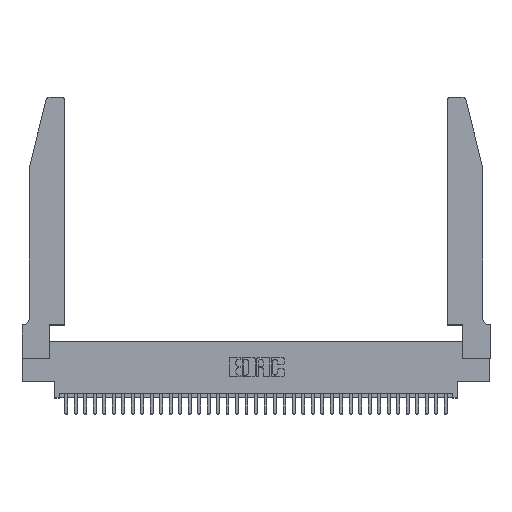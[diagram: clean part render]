
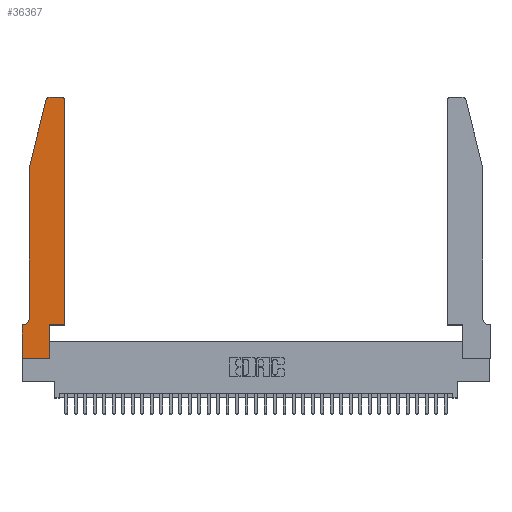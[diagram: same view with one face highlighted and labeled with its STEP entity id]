
A CAD part, top view. The second image highlights one B-rep face of the part: STEP entity #36367.
In plain terms, the highlighted planar face has unit normal (0, 0, 1).
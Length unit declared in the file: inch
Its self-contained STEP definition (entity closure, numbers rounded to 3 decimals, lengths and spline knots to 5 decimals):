
#19 = EDGE_LOOP ( 'NONE', ( #13343, #34293, #35894, #194, #32625, #27486, #5706, #4001, #19048, #23424, #12861, #13882 ) ) ;
#194 = ORIENTED_EDGE ( 'NONE', *, *, #6207, .T. ) ;
#359 = CIRCLE ( 'NONE', #16648, 0.03 ) ;
#873 = VECTOR ( 'NONE', #36660, 39.37008 ) ;
#877 = CARTESIAN_POINT ( 'NONE',  ( 0.4505, 0.35, 0.37 ) ) ;
#1088 = CARTESIAN_POINT ( 'NONE',  ( 0., 0.35, 0.37 ) ) ;
#2234 = VERTEX_POINT ( 'NONE', #5444 ) ;
#2669 = VECTOR ( 'NONE', #34483, 39.37008 ) ;
#3150 = CARTESIAN_POINT ( 'NONE',  ( 0., 0., 0.37 ) ) ;
#3686 = DIRECTION ( 'NONE',  ( 0., 1., 0. ) ) ;
#3735 = CARTESIAN_POINT ( 'NONE',  ( 0.0755, 0.42, 0.37 ) ) ;
#4001 = ORIENTED_EDGE ( 'NONE', *, *, #28637, .T. ) ;
#4124 = EDGE_CURVE ( 'NONE', #32632, #2234, #359, .T. ) ;
#4449 = CARTESIAN_POINT ( 'NONE',  ( 0.4505, 0.35, 0.37 ) ) ;
#4918 = VERTEX_POINT ( 'NONE', #33622 ) ;
#5171 = VERTEX_POINT ( 'NONE', #34726 ) ;
#5190 = VECTOR ( 'NONE', #11448, 39.37008 ) ;
#5444 = CARTESIAN_POINT ( 'NONE',  ( 0.4205, 2.75, 0.37 ) ) ;
#5706 = ORIENTED_EDGE ( 'NONE', *, *, #31145, .T. ) ;
#6207 = EDGE_CURVE ( 'NONE', #36018, #32110, #22789, .T. ) ;
#6238 = LINE ( 'NONE', #4449, #23822 ) ;
#6697 = CARTESIAN_POINT ( 'NONE',  ( 0.2865, 0.35, 0.37 ) ) ;
#6746 = LINE ( 'NONE', #19997, #2669 ) ;
#6781 = LINE ( 'NONE', #6697, #20322 ) ;
#6870 = DIRECTION ( 'NONE',  ( -0.239, -0.971, 0. ) ) ;
#7064 = DIRECTION ( 'NONE',  ( 0., 1., 0. ) ) ;
#7135 = DIRECTION ( 'NONE',  ( -1., 0., 0. ) ) ;
#7793 = DIRECTION ( 'NONE',  ( 0., 0., -1. ) ) ;
#8426 = VECTOR ( 'NONE', #12074, 39.37008 ) ;
#8512 = VERTEX_POINT ( 'NONE', #16217 ) ;
#8842 = CARTESIAN_POINT ( 'NONE',  ( 0.0755, 2., 0.37 ) ) ;
#9727 = LINE ( 'NONE', #29092, #8426 ) ;
#10071 = CARTESIAN_POINT ( 'NONE',  ( 0.4205, 2.72, 0.37 ) ) ;
#10494 = EDGE_CURVE ( 'NONE', #32110, #8512, #27063, .T. ) ;
#10648 = CARTESIAN_POINT ( 'NONE',  ( 0.25487, 2.72718, 0.37 ) ) ;
#11448 = DIRECTION ( 'NONE',  ( 1., 0., 0. ) ) ;
#11695 = LINE ( 'NONE', #29436, #17118 ) ;
#12074 = DIRECTION ( 'NONE',  ( 1., 0., 0. ) ) ;
#12132 = VERTEX_POINT ( 'NONE', #30353 ) ;
#12488 = VERTEX_POINT ( 'NONE', #28299 ) ;
#12534 = AXIS2_PLACEMENT_3D ( 'NONE', #33241, #13338, #36126 ) ;
#12861 = ORIENTED_EDGE ( 'NONE', *, *, #32862, .T. ) ;
#12865 = CARTESIAN_POINT ( 'NONE',  ( 0.0755, 2., 0.37 ) ) ;
#12996 = DIRECTION ( 'NONE',  ( 0., 0., 1. ) ) ;
#13338 = DIRECTION ( 'NONE',  ( 0., 0., 1. ) ) ;
#13343 = ORIENTED_EDGE ( 'NONE', *, *, #27340, .T. ) ;
#13882 = ORIENTED_EDGE ( 'NONE', *, *, #4124, .T. ) ;
#15532 = AXIS2_PLACEMENT_3D ( 'NONE', #22175, #7793, #24932 ) ;
#15855 = EDGE_CURVE ( 'NONE', #12488, #22731, #22346, .T. ) ;
#16217 = CARTESIAN_POINT ( 'NONE',  ( 0.0055, 0.35, 0.37 ) ) ;
#16265 = EDGE_CURVE ( 'NONE', #8512, #5171, #34913, .T. ) ;
#16537 = CIRCLE ( 'NONE', #12534, 0.03 ) ;
#16648 = AXIS2_PLACEMENT_3D ( 'NONE', #10071, #30124, #33539 ) ;
#17118 = VECTOR ( 'NONE', #6870, 39.37008 ) ;
#17924 = CARTESIAN_POINT ( 'NONE',  ( 0.4505, 2.72, 0.37 ) ) ;
#18382 = VERTEX_POINT ( 'NONE', #25051 ) ;
#18395 = EDGE_CURVE ( 'NONE', #4918, #32265, #16537, .T. ) ;
#19048 = ORIENTED_EDGE ( 'NONE', *, *, #26976, .T. ) ;
#19062 = FACE_OUTER_BOUND ( 'NONE', #19, .T. ) ;
#19161 = VECTOR ( 'NONE', #7135, 39.37008 ) ;
#19997 = CARTESIAN_POINT ( 'NONE',  ( 0.2605, 2.75, 0.37 ) ) ;
#20322 = VECTOR ( 'NONE', #3686, 39.37008 ) ;
#21280 = CARTESIAN_POINT ( 'NONE',  ( 0.0755, 0.35, 0.37 ) ) ;
#22175 = CARTESIAN_POINT ( 'NONE',  ( 0.0055, 0.42, 0.37 ) ) ;
#22346 = LINE ( 'NONE', #25324, #5190 ) ;
#22731 = VERTEX_POINT ( 'NONE', #877 ) ;
#22789 = LINE ( 'NONE', #12865, #28625 ) ;
#23424 = ORIENTED_EDGE ( 'NONE', *, *, #15855, .T. ) ;
#23822 = VECTOR ( 'NONE', #7064, 39.37008 ) ;
#24459 = PLANE ( 'NONE',  #34054 ) ;
#24932 = DIRECTION ( 'NONE',  ( -1., 0., 0. ) ) ;
#25051 = CARTESIAN_POINT ( 'NONE',  ( 0., 0., 0.37 ) ) ;
#25324 = CARTESIAN_POINT ( 'NONE',  ( 0.4505, 0.35, 0.37 ) ) ;
#26853 = DIRECTION ( 'NONE',  ( 1., 0., 0. ) ) ;
#26976 = EDGE_CURVE ( 'NONE', #12132, #12488, #6781, .T. ) ;
#27063 = CIRCLE ( 'NONE', #15532, 0.07 ) ;
#27340 = EDGE_CURVE ( 'NONE', #2234, #4918, #6746, .T. ) ;
#27486 = ORIENTED_EDGE ( 'NONE', *, *, #16265, .T. ) ;
#28299 = CARTESIAN_POINT ( 'NONE',  ( 0.2865, 0.35, 0.37 ) ) ;
#28625 = VECTOR ( 'NONE', #30864, 39.37008 ) ;
#28637 = EDGE_CURVE ( 'NONE', #18382, #12132, #9727, .T. ) ;
#29092 = CARTESIAN_POINT ( 'NONE',  ( 0., 0., 0.37 ) ) ;
#29436 = CARTESIAN_POINT ( 'NONE',  ( 0.0755, 2., 0.37 ) ) ;
#30124 = DIRECTION ( 'NONE',  ( 0., 0., 1. ) ) ;
#30353 = CARTESIAN_POINT ( 'NONE',  ( 0.2865, 0., 0.37 ) ) ;
#30864 = DIRECTION ( 'NONE',  ( 0., -1., 0. ) ) ;
#31145 = EDGE_CURVE ( 'NONE', #5171, #18382, #32018, .T. ) ;
#32018 = LINE ( 'NONE', #3150, #873 ) ;
#32073 = EDGE_CURVE ( 'NONE', #32265, #36018, #11695, .T. ) ;
#32110 = VERTEX_POINT ( 'NONE', #3735 ) ;
#32265 = VERTEX_POINT ( 'NONE', #10648 ) ;
#32625 = ORIENTED_EDGE ( 'NONE', *, *, #10494, .T. ) ;
#32632 = VERTEX_POINT ( 'NONE', #17924 ) ;
#32862 = EDGE_CURVE ( 'NONE', #22731, #32632, #6238, .T. ) ;
#33241 = CARTESIAN_POINT ( 'NONE',  ( 0.284, 2.72, 0.37 ) ) ;
#33539 = DIRECTION ( 'NONE',  ( 1., 0., 0. ) ) ;
#33622 = CARTESIAN_POINT ( 'NONE',  ( 0.284, 2.75, 0.37 ) ) ;
#34054 = AXIS2_PLACEMENT_3D ( 'NONE', #1088, #12996, #26853 ) ;
#34293 = ORIENTED_EDGE ( 'NONE', *, *, #18395, .T. ) ;
#34483 = DIRECTION ( 'NONE',  ( -1., 0., 0. ) ) ;
#34726 = CARTESIAN_POINT ( 'NONE',  ( 0., 0.35, 0.37 ) ) ;
#34913 = LINE ( 'NONE', #21280, #19161 ) ;
#35894 = ORIENTED_EDGE ( 'NONE', *, *, #32073, .T. ) ;
#36018 = VERTEX_POINT ( 'NONE', #8842 ) ;
#36126 = DIRECTION ( 'NONE',  ( 1., 0., 0. ) ) ;
#36367 = ADVANCED_FACE ( 'NONE', ( #19062 ), #24459, .T. ) ;
#36660 = DIRECTION ( 'NONE',  ( 0., -1., 0. ) ) ;
